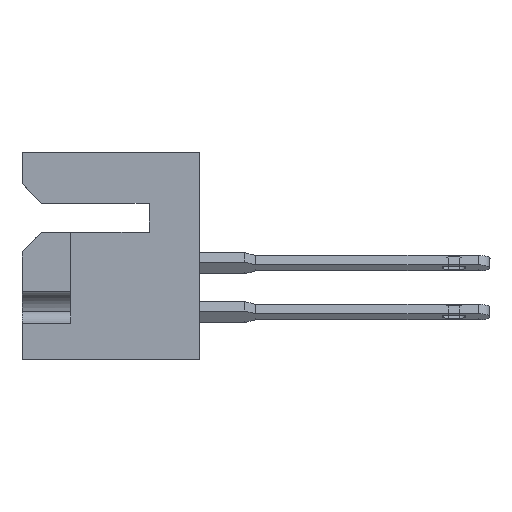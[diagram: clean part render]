
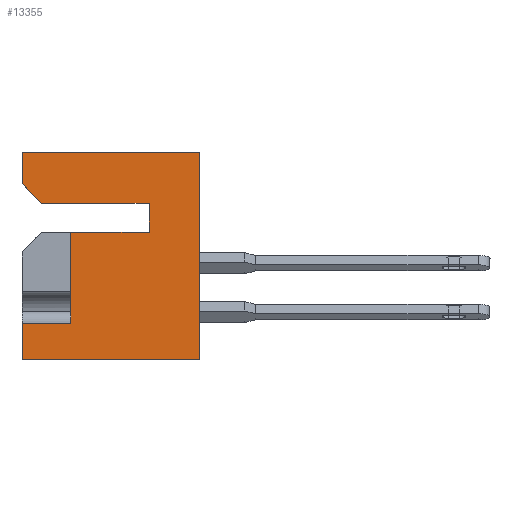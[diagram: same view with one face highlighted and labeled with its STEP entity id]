
A CAD part, left-side view. The second image highlights one B-rep face of the part: STEP entity #13355.
In plain terms, the highlighted planar face has unit normal (-1, 0, 0).
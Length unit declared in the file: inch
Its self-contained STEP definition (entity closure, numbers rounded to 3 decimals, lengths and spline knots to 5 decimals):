
#376 = ORIENTED_EDGE ( 'NONE', *, *, #26908, .F. ) ;
#580 = VERTEX_POINT ( 'NONE', #6248 ) ;
#944 = CARTESIAN_POINT ( 'NONE',  ( 0., 0.453, 0. ) ) ;
#1310 = VERTEX_POINT ( 'NONE', #26403 ) ;
#1436 = VERTEX_POINT ( 'NONE', #22190 ) ;
#1645 = EDGE_CURVE ( 'NONE', #5893, #11007, #17692, .T. ) ;
#1944 = ORIENTED_EDGE ( 'NONE', *, *, #19616, .T. ) ;
#2764 = EDGE_CURVE ( 'NONE', #11007, #19683, #16291, .T. ) ;
#2996 = DIRECTION ( 'NONE',  ( 0., -1., 0. ) ) ;
#3029 = VECTOR ( 'NONE', #25297, 39.37008 ) ;
#3180 = LINE ( 'NONE', #9798, #19369 ) ;
#3601 = ORIENTED_EDGE ( 'NONE', *, *, #22560, .T. ) ;
#3860 = DIRECTION ( 'NONE',  ( 0., 0., 1. ) ) ;
#3935 = VERTEX_POINT ( 'NONE', #15523 ) ;
#4157 = DIRECTION ( 'NONE',  ( 0., 0., -1. ) ) ;
#4184 = LINE ( 'NONE', #17610, #10456 ) ;
#4329 = EDGE_CURVE ( 'NONE', #19994, #11365, #17651, .T. ) ;
#4932 = CARTESIAN_POINT ( 'NONE',  ( 0., 0.128, -0.131 ) ) ;
#5324 = LINE ( 'NONE', #19175, #13590 ) ;
#5434 = DIRECTION ( 'NONE',  ( 0., -0.707, -0.707 ) ) ;
#5486 = CARTESIAN_POINT ( 'NONE',  ( 0., 0.453, 0. ) ) ;
#5893 = VERTEX_POINT ( 'NONE', #7036 ) ;
#6202 = PLANE ( 'NONE',  #7248 ) ;
#6248 = CARTESIAN_POINT ( 'NONE',  ( 0., 0.453, -0.531 ) ) ;
#6602 = DIRECTION ( 'NONE',  ( 0., -1., 0. ) ) ;
#6640 = ORIENTED_EDGE ( 'NONE', *, *, #19476, .T. ) ;
#7036 = CARTESIAN_POINT ( 'NONE',  ( 0., 0.453, -0.081 ) ) ;
#7198 = CARTESIAN_POINT ( 'NONE',  ( 0., 0.128, -0.131 ) ) ;
#7248 = AXIS2_PLACEMENT_3D ( 'NONE', #12375, #12470, #4157 ) ;
#7965 = CARTESIAN_POINT ( 'NONE',  ( 0., 0., 0. ) ) ;
#8298 = ORIENTED_EDGE ( 'NONE', *, *, #1645, .F. ) ;
#8673 = VECTOR ( 'NONE', #25614, 39.37008 ) ;
#9045 = ORIENTED_EDGE ( 'NONE', *, *, #10316, .F. ) ;
#9330 = VECTOR ( 'NONE', #6602, 39.37008 ) ;
#9798 = CARTESIAN_POINT ( 'NONE',  ( 0., 0.128, -0.205 ) ) ;
#9981 = EDGE_CURVE ( 'NONE', #27034, #19994, #24620, .T. ) ;
#9986 = DIRECTION ( 'NONE',  ( 0., 1., 0. ) ) ;
#10144 = LINE ( 'NONE', #26552, #20729 ) ;
#10316 = EDGE_CURVE ( 'NONE', #580, #1310, #4184, .T. ) ;
#10456 = VECTOR ( 'NONE', #21855, 39.37008 ) ;
#10777 = CARTESIAN_POINT ( 'NONE',  ( 0., 0.328, -0.437 ) ) ;
#11007 = VERTEX_POINT ( 'NONE', #944 ) ;
#11365 = VERTEX_POINT ( 'NONE', #14792 ) ;
#11719 = ORIENTED_EDGE ( 'NONE', *, *, #13472, .T. ) ;
#11833 = VECTOR ( 'NONE', #5434, 39.37008 ) ;
#12251 = EDGE_LOOP ( 'NONE', ( #11719, #9045, #6640, #18304, #17303, #8298, #3601, #18971, #21798, #1944, #376 ) ) ;
#12375 = CARTESIAN_POINT ( 'NONE',  ( 0., 0.453, 0. ) ) ;
#12470 = DIRECTION ( 'NONE',  ( 1., 0., 0. ) ) ;
#13355 = ADVANCED_FACE ( 'NONE', ( #20245 ), #6202, .F. ) ;
#13472 = EDGE_CURVE ( 'NONE', #1436, #1310, #23232, .T. ) ;
#13590 = VECTOR ( 'NONE', #23357, 39.37008 ) ;
#13964 = EDGE_CURVE ( 'NONE', #3935, #19683, #19229, .T. ) ;
#14723 = VECTOR ( 'NONE', #3860, 39.37008 ) ;
#14792 = CARTESIAN_POINT ( 'NONE',  ( 0., 0.403, -0.131 ) ) ;
#15395 = CARTESIAN_POINT ( 'NONE',  ( 0., 0.128, -0.205 ) ) ;
#15523 = CARTESIAN_POINT ( 'NONE',  ( 0., 0., -0.531 ) ) ;
#15809 = LINE ( 'NONE', #16152, #11833 ) ;
#16152 = CARTESIAN_POINT ( 'NONE',  ( 0., 0.403, -0.131 ) ) ;
#16291 = LINE ( 'NONE', #27305, #9330 ) ;
#16606 = CARTESIAN_POINT ( 'NONE',  ( 0., 0., 0. ) ) ;
#16620 = VERTEX_POINT ( 'NONE', #21984 ) ;
#17303 = ORIENTED_EDGE ( 'NONE', *, *, #2764, .F. ) ;
#17610 = CARTESIAN_POINT ( 'NONE',  ( 0., 0.453, 0. ) ) ;
#17651 = LINE ( 'NONE', #4932, #18968 ) ;
#17671 = DIRECTION ( 'NONE',  ( 0., 1., 0. ) ) ;
#17692 = LINE ( 'NONE', #5486, #26950 ) ;
#18304 = ORIENTED_EDGE ( 'NONE', *, *, #13964, .T. ) ;
#18968 = VECTOR ( 'NONE', #17671, 39.37008 ) ;
#18971 = ORIENTED_EDGE ( 'NONE', *, *, #4329, .F. ) ;
#19175 = CARTESIAN_POINT ( 'NONE',  ( 0., 0.328, -0.205 ) ) ;
#19229 = LINE ( 'NONE', #16606, #3029 ) ;
#19369 = VECTOR ( 'NONE', #9986, 39.37008 ) ;
#19476 = EDGE_CURVE ( 'NONE', #580, #3935, #10144, .T. ) ;
#19616 = EDGE_CURVE ( 'NONE', #27034, #16620, #3180, .T. ) ;
#19683 = VERTEX_POINT ( 'NONE', #7965 ) ;
#19994 = VERTEX_POINT ( 'NONE', #7198 ) ;
#20245 = FACE_OUTER_BOUND ( 'NONE', #12251, .T. ) ;
#20729 = VECTOR ( 'NONE', #2996, 39.37008 ) ;
#21798 = ORIENTED_EDGE ( 'NONE', *, *, #9981, .F. ) ;
#21855 = DIRECTION ( 'NONE',  ( 0., 0., 1. ) ) ;
#21984 = CARTESIAN_POINT ( 'NONE',  ( 0., 0.328, -0.205 ) ) ;
#22127 = DIRECTION ( 'NONE',  ( 0., 0., 1. ) ) ;
#22190 = CARTESIAN_POINT ( 'NONE',  ( 0., 0.328, -0.437 ) ) ;
#22560 = EDGE_CURVE ( 'NONE', #5893, #11365, #15809, .T. ) ;
#23232 = LINE ( 'NONE', #10777, #8673 ) ;
#23357 = DIRECTION ( 'NONE',  ( 0., 0., 1. ) ) ;
#24620 = LINE ( 'NONE', #27241, #14723 ) ;
#25297 = DIRECTION ( 'NONE',  ( 0., 0., 1. ) ) ;
#25614 = DIRECTION ( 'NONE',  ( 0., 1., 0. ) ) ;
#26403 = CARTESIAN_POINT ( 'NONE',  ( 0., 0.453, -0.437 ) ) ;
#26552 = CARTESIAN_POINT ( 'NONE',  ( 0., 0.453, -0.531 ) ) ;
#26908 = EDGE_CURVE ( 'NONE', #1436, #16620, #5324, .T. ) ;
#26950 = VECTOR ( 'NONE', #22127, 39.37008 ) ;
#27034 = VERTEX_POINT ( 'NONE', #15395 ) ;
#27241 = CARTESIAN_POINT ( 'NONE',  ( 0., 0.128, -0.131 ) ) ;
#27305 = CARTESIAN_POINT ( 'NONE',  ( 0., 0.453, 0. ) ) ;
